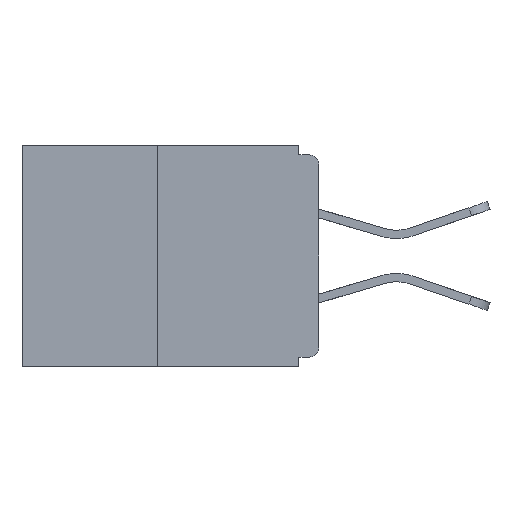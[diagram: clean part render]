
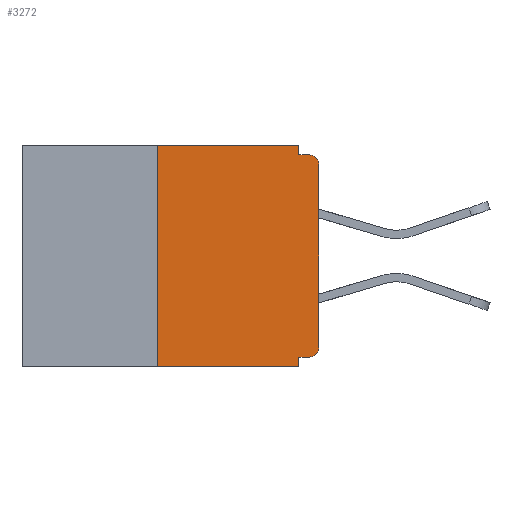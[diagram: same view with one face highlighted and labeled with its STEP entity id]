
A CAD part, left-side view. The second image highlights one B-rep face of the part: STEP entity #3272.
In plain terms, the highlighted planar face has unit normal (-1, 0, 0).
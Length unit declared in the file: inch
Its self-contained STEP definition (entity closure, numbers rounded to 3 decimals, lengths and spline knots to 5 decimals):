
#55 = DIRECTION ( 'NONE',  ( 0., 1., 0. ) ) ;
#296 = LINE ( 'NONE', #1827, #16778 ) ;
#308 = DIRECTION ( 'NONE',  ( -1., 0., 0. ) ) ;
#372 = CARTESIAN_POINT ( 'NONE',  ( 0., 0., -0.313 ) ) ;
#853 = AXIS2_PLACEMENT_3D ( 'NONE', #6387, #308, #3267 ) ;
#1479 = VERTEX_POINT ( 'NONE', #5012 ) ;
#1580 = AXIS2_PLACEMENT_3D ( 'NONE', #8025, #9451, #18535 ) ;
#1827 = CARTESIAN_POINT ( 'NONE',  ( 0., 0.031, -0.343 ) ) ;
#2320 = DIRECTION ( 'NONE',  ( -1., 0., 0. ) ) ;
#2476 = ORIENTED_EDGE ( 'NONE', *, *, #6658, .F. ) ;
#3267 = DIRECTION ( 'NONE',  ( 0., 0., -1. ) ) ;
#3272 = ADVANCED_FACE ( 'NONE', ( #19146 ), #11127, .F. ) ;
#3322 = ORIENTED_EDGE ( 'NONE', *, *, #17937, .T. ) ;
#3553 = VERTEX_POINT ( 'NONE', #8775 ) ;
#3917 = VECTOR ( 'NONE', #5866, 39.37008 ) ;
#4008 = EDGE_CURVE ( 'NONE', #17520, #1479, #12523, .T. ) ;
#4420 = CARTESIAN_POINT ( 'NONE',  ( 0., 0., -0.328 ) ) ;
#4492 = CARTESIAN_POINT ( 'NONE',  ( 0., 0., -0.015 ) ) ;
#4630 = CARTESIAN_POINT ( 'NONE',  ( 0., 0.46, 0. ) ) ;
#4732 = LINE ( 'NONE', #4420, #5901 ) ;
#5012 = CARTESIAN_POINT ( 'NONE',  ( 0., 0.015, -0.015 ) ) ;
#5333 = DIRECTION ( 'NONE',  ( 0., 0., 1. ) ) ;
#5390 = ORIENTED_EDGE ( 'NONE', *, *, #8372, .F. ) ;
#5728 = EDGE_CURVE ( 'NONE', #12872, #17520, #14122, .T. ) ;
#5765 = VECTOR ( 'NONE', #12010, 39.37008 ) ;
#5866 = DIRECTION ( 'NONE',  ( 0., -1., 0. ) ) ;
#5901 = VECTOR ( 'NONE', #55, 39.37008 ) ;
#5971 = CARTESIAN_POINT ( 'NONE',  ( 0., 0.031, -0.328 ) ) ;
#6387 = CARTESIAN_POINT ( 'NONE',  ( 0., 0.015, -0.03 ) ) ;
#6440 = VECTOR ( 'NONE', #5333, 39.37008 ) ;
#6643 = CIRCLE ( 'NONE', #853, 0.015 ) ;
#6658 = EDGE_CURVE ( 'NONE', #9177, #3553, #6899, .T. ) ;
#6899 = LINE ( 'NONE', #8348, #6440 ) ;
#7117 = EDGE_CURVE ( 'NONE', #8540, #1479, #6643, .T. ) ;
#7337 = CARTESIAN_POINT ( 'NONE',  ( 0., 0.031, 0. ) ) ;
#7406 = ORIENTED_EDGE ( 'NONE', *, *, #15558, .F. ) ;
#7673 = CARTESIAN_POINT ( 'NONE',  ( 0., 0.031, 0. ) ) ;
#8025 = CARTESIAN_POINT ( 'NONE',  ( 0., 0.46, 0. ) ) ;
#8177 = EDGE_CURVE ( 'NONE', #15989, #8540, #12164, .T. ) ;
#8348 = CARTESIAN_POINT ( 'NONE',  ( 0., 0.25, 0. ) ) ;
#8372 = EDGE_CURVE ( 'NONE', #14428, #13270, #4732, .T. ) ;
#8540 = VERTEX_POINT ( 'NONE', #11287 ) ;
#8775 = CARTESIAN_POINT ( 'NONE',  ( 0., 0.25, 0. ) ) ;
#8885 = CARTESIAN_POINT ( 'NONE',  ( 0., 0., 0. ) ) ;
#9149 = LINE ( 'NONE', #4630, #14534 ) ;
#9177 = VERTEX_POINT ( 'NONE', #9720 ) ;
#9451 = DIRECTION ( 'NONE',  ( 1., 0., 0. ) ) ;
#9720 = CARTESIAN_POINT ( 'NONE',  ( 0., 0.25, -0.343 ) ) ;
#9805 = DIRECTION ( 'NONE',  ( 0., -1., 0. ) ) ;
#11004 = CARTESIAN_POINT ( 'NONE',  ( 0., 0.031, -0.015 ) ) ;
#11127 = PLANE ( 'NONE',  #1580 ) ;
#11164 = EDGE_CURVE ( 'NONE', #13270, #17101, #296, .T. ) ;
#11287 = CARTESIAN_POINT ( 'NONE',  ( 0., 0., -0.03 ) ) ;
#11464 = VECTOR ( 'NONE', #11920, 39.37008 ) ;
#11555 = AXIS2_PLACEMENT_3D ( 'NONE', #18658, #2320, #15682 ) ;
#11920 = DIRECTION ( 'NONE',  ( 0., 0., 1. ) ) ;
#12010 = DIRECTION ( 'NONE',  ( 0., 0., -1. ) ) ;
#12164 = LINE ( 'NONE', #8885, #11464 ) ;
#12436 = ORIENTED_EDGE ( 'NONE', *, *, #4008, .F. ) ;
#12523 = LINE ( 'NONE', #4492, #3917 ) ;
#12872 = VERTEX_POINT ( 'NONE', #7673 ) ;
#13259 = ORIENTED_EDGE ( 'NONE', *, *, #5728, .F. ) ;
#13270 = VERTEX_POINT ( 'NONE', #5971 ) ;
#13360 = CARTESIAN_POINT ( 'NONE',  ( 0., 0.015, -0.328 ) ) ;
#13542 = ORIENTED_EDGE ( 'NONE', *, *, #17111, .T. ) ;
#13563 = ORIENTED_EDGE ( 'NONE', *, *, #11164, .F. ) ;
#13791 = EDGE_LOOP ( 'NONE', ( #7406, #2476, #13542, #13563, #5390, #3322, #16450, #16802, #12436, #13259 ) ) ;
#14022 = CARTESIAN_POINT ( 'NONE',  ( 0., 0.031, -0.343 ) ) ;
#14122 = LINE ( 'NONE', #7337, #5765 ) ;
#14428 = VERTEX_POINT ( 'NONE', #13360 ) ;
#14534 = VECTOR ( 'NONE', #18063, 39.37008 ) ;
#15167 = DIRECTION ( 'NONE',  ( 0., 0., -1. ) ) ;
#15558 = EDGE_CURVE ( 'NONE', #3553, #12872, #9149, .T. ) ;
#15656 = CARTESIAN_POINT ( 'NONE',  ( 0., 0.46, -0.343 ) ) ;
#15682 = DIRECTION ( 'NONE',  ( 0., 0., -1. ) ) ;
#15890 = CIRCLE ( 'NONE', #11555, 0.015 ) ;
#15989 = VERTEX_POINT ( 'NONE', #372 ) ;
#16450 = ORIENTED_EDGE ( 'NONE', *, *, #8177, .T. ) ;
#16613 = LINE ( 'NONE', #15656, #18473 ) ;
#16778 = VECTOR ( 'NONE', #15167, 39.37008 ) ;
#16802 = ORIENTED_EDGE ( 'NONE', *, *, #7117, .T. ) ;
#17101 = VERTEX_POINT ( 'NONE', #14022 ) ;
#17111 = EDGE_CURVE ( 'NONE', #9177, #17101, #16613, .T. ) ;
#17520 = VERTEX_POINT ( 'NONE', #11004 ) ;
#17937 = EDGE_CURVE ( 'NONE', #14428, #15989, #15890, .T. ) ;
#18063 = DIRECTION ( 'NONE',  ( 0., -1., 0. ) ) ;
#18473 = VECTOR ( 'NONE', #9805, 39.37008 ) ;
#18535 = DIRECTION ( 'NONE',  ( 0., 0., -1. ) ) ;
#18658 = CARTESIAN_POINT ( 'NONE',  ( 0., 0.015, -0.313 ) ) ;
#19146 = FACE_OUTER_BOUND ( 'NONE', #13791, .T. ) ;
